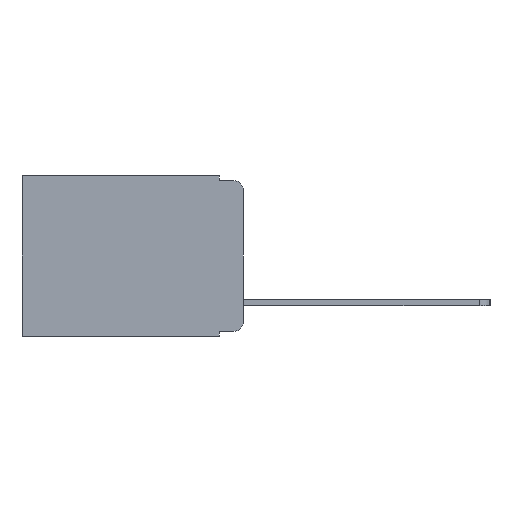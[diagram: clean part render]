
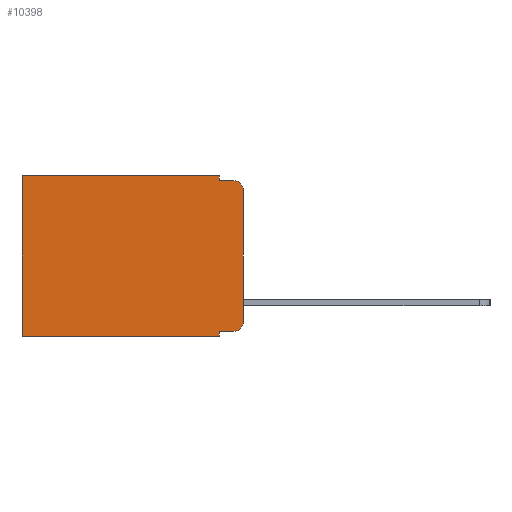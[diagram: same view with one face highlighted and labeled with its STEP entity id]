
A CAD part, left-side view. The second image highlights one B-rep face of the part: STEP entity #10398.
In plain terms, the highlighted planar face has unit normal (-1, 0, 0).
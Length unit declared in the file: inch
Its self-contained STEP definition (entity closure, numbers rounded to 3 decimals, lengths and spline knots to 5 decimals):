
#1425 = VERTEX_POINT ( 'NONE', #11835 ) ;
#1466 = AXIS2_PLACEMENT_3D ( 'NONE', #15582, #16845, #9044 ) ;
#1538 = LINE ( 'NONE', #9707, #9281 ) ;
#1871 = EDGE_CURVE ( 'NONE', #8496, #8544, #17056, .T. ) ;
#2226 = CARTESIAN_POINT ( 'NONE',  ( 0.298, 0., -0.313 ) ) ;
#2355 = EDGE_CURVE ( 'NONE', #12649, #5845, #6069, .T. ) ;
#2374 = VERTEX_POINT ( 'NONE', #12773 ) ;
#2566 = DIRECTION ( 'NONE',  ( 0., -1., 0. ) ) ;
#2631 = VERTEX_POINT ( 'NONE', #11459 ) ;
#2738 = EDGE_CURVE ( 'NONE', #2374, #13354, #7372, .T. ) ;
#2842 = DIRECTION ( 'NONE',  ( -1., 0., 0. ) ) ;
#3333 = CARTESIAN_POINT ( 'NONE',  ( 0.298, 0.02, -0.03 ) ) ;
#3644 = EDGE_CURVE ( 'NONE', #1425, #7158, #6835, .T. ) ;
#3680 = FACE_OUTER_BOUND ( 'NONE', #9336, .T. ) ;
#4022 = LINE ( 'NONE', #11782, #6112 ) ;
#4925 = EDGE_CURVE ( 'NONE', #12649, #2631, #7631, .T. ) ;
#4945 = CARTESIAN_POINT ( 'NONE',  ( 0.298, 0., 0. ) ) ;
#5368 = ORIENTED_EDGE ( 'NONE', *, *, #11051, .F. ) ;
#5845 = VERTEX_POINT ( 'NONE', #12119 ) ;
#5951 = AXIS2_PLACEMENT_3D ( 'NONE', #14296, #14316, #17473 ) ;
#6002 = ORIENTED_EDGE ( 'NONE', *, *, #3644, .T. ) ;
#6069 = LINE ( 'NONE', #9129, #15864 ) ;
#6098 = CARTESIAN_POINT ( 'NONE',  ( 0.298, 0.02, -0.01 ) ) ;
#6112 = VECTOR ( 'NONE', #6472, 39.37008 ) ;
#6233 = VECTOR ( 'NONE', #14435, 39.37008 ) ;
#6257 = PLANE ( 'NONE',  #1466 ) ;
#6472 = DIRECTION ( 'NONE',  ( 0., 0., -1. ) ) ;
#6496 = ORIENTED_EDGE ( 'NONE', *, *, #11799, .F. ) ;
#6535 = VECTOR ( 'NONE', #15562, 39.37008 ) ;
#6835 = CIRCLE ( 'NONE', #16551, 0.02 ) ;
#7012 = ORIENTED_EDGE ( 'NONE', *, *, #2355, .F. ) ;
#7158 = VERTEX_POINT ( 'NONE', #6098 ) ;
#7175 = DIRECTION ( 'NONE',  ( 0., 1., 0. ) ) ;
#7372 = CIRCLE ( 'NONE', #5951, 0.02 ) ;
#7471 = ORIENTED_EDGE ( 'NONE', *, *, #4925, .T. ) ;
#7631 = LINE ( 'NONE', #12503, #14305 ) ;
#7794 = ORIENTED_EDGE ( 'NONE', *, *, #13903, .T. ) ;
#7972 = ORIENTED_EDGE ( 'NONE', *, *, #1871, .F. ) ;
#8384 = ORIENTED_EDGE ( 'NONE', *, *, #11248, .F. ) ;
#8496 = VERTEX_POINT ( 'NONE', #10888 ) ;
#8544 = VERTEX_POINT ( 'NONE', #17444 ) ;
#8818 = ORIENTED_EDGE ( 'NONE', *, *, #17640, .T. ) ;
#9044 = DIRECTION ( 'NONE',  ( 0., 0., -1. ) ) ;
#9129 = CARTESIAN_POINT ( 'NONE',  ( 0.298, 0.051, 0. ) ) ;
#9220 = ORIENTED_EDGE ( 'NONE', *, *, #2738, .T. ) ;
#9281 = VECTOR ( 'NONE', #2566, 39.37008 ) ;
#9336 = EDGE_LOOP ( 'NONE', ( #5368, #6002, #6496, #7012, #7471, #7794, #7972, #8384, #8818, #9220 ) ) ;
#9707 = CARTESIAN_POINT ( 'NONE',  ( 0.298, 0.051, -0.333 ) ) ;
#10083 = LINE ( 'NONE', #17665, #16601 ) ;
#10257 = LINE ( 'NONE', #10936, #13372 ) ;
#10296 = VERTEX_POINT ( 'NONE', #12808 ) ;
#10398 = ADVANCED_FACE ( 'NONE', ( #3680 ), #6257, .F. ) ;
#10435 = CARTESIAN_POINT ( 'NONE',  ( 0.298, 0.051, 0. ) ) ;
#10888 = CARTESIAN_POINT ( 'NONE',  ( 0.298, 0.051, -0.343 ) ) ;
#10936 = CARTESIAN_POINT ( 'NONE',  ( 0.298, 0.051, -0.01 ) ) ;
#11051 = EDGE_CURVE ( 'NONE', #1425, #13354, #13407, .T. ) ;
#11052 = CARTESIAN_POINT ( 'NONE',  ( 0.298, 0., -0.343 ) ) ;
#11248 = EDGE_CURVE ( 'NONE', #10296, #8496, #10083, .T. ) ;
#11459 = CARTESIAN_POINT ( 'NONE',  ( 0.298, 0.473, 0. ) ) ;
#11782 = CARTESIAN_POINT ( 'NONE',  ( 0.298, 0.473, 0. ) ) ;
#11799 = EDGE_CURVE ( 'NONE', #5845, #7158, #10257, .T. ) ;
#11835 = CARTESIAN_POINT ( 'NONE',  ( 0.298, 0., -0.03 ) ) ;
#12119 = CARTESIAN_POINT ( 'NONE',  ( 0.298, 0.051, -0.01 ) ) ;
#12254 = DIRECTION ( 'NONE',  ( 0., -1., 0. ) ) ;
#12434 = DIRECTION ( 'NONE',  ( 0., 0., -1. ) ) ;
#12503 = CARTESIAN_POINT ( 'NONE',  ( 0.298, 0., 0. ) ) ;
#12649 = VERTEX_POINT ( 'NONE', #10435 ) ;
#12773 = CARTESIAN_POINT ( 'NONE',  ( 0.298, 0.02, -0.333 ) ) ;
#12808 = CARTESIAN_POINT ( 'NONE',  ( 0.298, 0.051, -0.333 ) ) ;
#13273 = DIRECTION ( 'NONE',  ( 0., 0., -1. ) ) ;
#13354 = VERTEX_POINT ( 'NONE', #2226 ) ;
#13372 = VECTOR ( 'NONE', #12254, 39.37008 ) ;
#13407 = LINE ( 'NONE', #4945, #6233 ) ;
#13903 = EDGE_CURVE ( 'NONE', #2631, #8544, #4022, .T. ) ;
#14296 = CARTESIAN_POINT ( 'NONE',  ( 0.298, 0.02, -0.313 ) ) ;
#14305 = VECTOR ( 'NONE', #7175, 39.37008 ) ;
#14316 = DIRECTION ( 'NONE',  ( -1., 0., 0. ) ) ;
#14435 = DIRECTION ( 'NONE',  ( 0., 0., -1. ) ) ;
#14617 = DIRECTION ( 'NONE',  ( 0., 0., -1. ) ) ;
#15562 = DIRECTION ( 'NONE',  ( 0., 1., 0. ) ) ;
#15582 = CARTESIAN_POINT ( 'NONE',  ( 0.298, 0., 0. ) ) ;
#15864 = VECTOR ( 'NONE', #13273, 39.37008 ) ;
#16551 = AXIS2_PLACEMENT_3D ( 'NONE', #3333, #2842, #14617 ) ;
#16601 = VECTOR ( 'NONE', #12434, 39.37008 ) ;
#16845 = DIRECTION ( 'NONE',  ( 1., 0., 0. ) ) ;
#17056 = LINE ( 'NONE', #11052, #6535 ) ;
#17444 = CARTESIAN_POINT ( 'NONE',  ( 0.298, 0.473, -0.343 ) ) ;
#17473 = DIRECTION ( 'NONE',  ( 0., 0., -1. ) ) ;
#17640 = EDGE_CURVE ( 'NONE', #10296, #2374, #1538, .T. ) ;
#17665 = CARTESIAN_POINT ( 'NONE',  ( 0.298, 0.051, 0. ) ) ;
